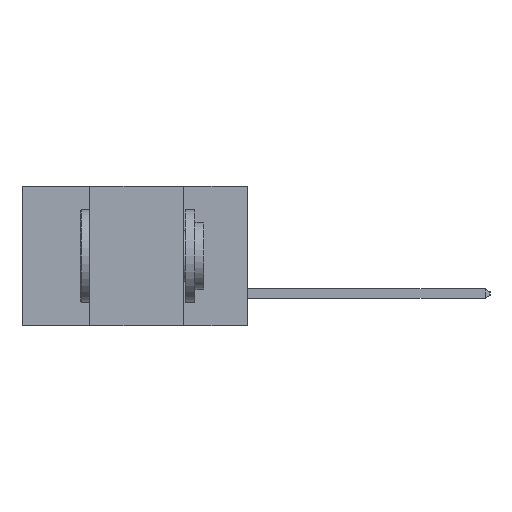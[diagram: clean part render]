
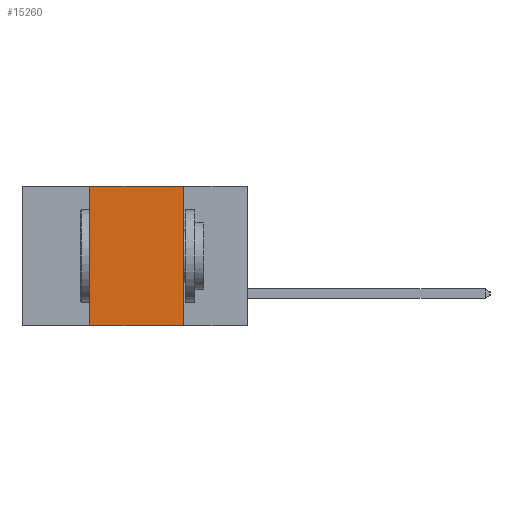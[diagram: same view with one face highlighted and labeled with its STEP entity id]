
A CAD part, left-side view. The second image highlights one B-rep face of the part: STEP entity #15260.
In plain terms, the highlighted planar face has unit normal (-1, 0, 0).
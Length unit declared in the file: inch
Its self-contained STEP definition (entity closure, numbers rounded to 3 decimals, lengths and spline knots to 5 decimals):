
#165 = CARTESIAN_POINT ( 'NONE',  ( 0., 0.6, -0.37 ) ) ;
#484 = CARTESIAN_POINT ( 'NONE',  ( 0., 0.42, -0.37 ) ) ;
#846 = CARTESIAN_POINT ( 'NONE',  ( 0., 0.6, 0. ) ) ;
#997 = VERTEX_POINT ( 'NONE', #6950 ) ;
#1227 = FACE_OUTER_BOUND ( 'NONE', #2528, .T. ) ;
#1617 = DIRECTION ( 'NONE',  ( 0., 0., -1. ) ) ;
#2177 = DIRECTION ( 'NONE',  ( 0., 0., -1. ) ) ;
#2320 = VERTEX_POINT ( 'NONE', #14089 ) ;
#2423 = DIRECTION ( 'NONE',  ( 0., -1., 0. ) ) ;
#2528 = EDGE_LOOP ( 'NONE', ( #11863, #14733, #8106, #14345 ) ) ;
#3344 = CARTESIAN_POINT ( 'NONE',  ( 0., 0.17, 0. ) ) ;
#6248 = CARTESIAN_POINT ( 'NONE',  ( 0., 0.6, 0. ) ) ;
#6489 = AXIS2_PLACEMENT_3D ( 'NONE', #846, #9815, #2177 ) ;
#6950 = CARTESIAN_POINT ( 'NONE',  ( 0., 0.42, 0. ) ) ;
#7304 = EDGE_CURVE ( 'NONE', #997, #10153, #13862, .T. ) ;
#7731 = VECTOR ( 'NONE', #1617, 39.37008 ) ;
#7892 = DIRECTION ( 'NONE',  ( 0., -1., 0. ) ) ;
#8106 = ORIENTED_EDGE ( 'NONE', *, *, #13539, .F. ) ;
#8115 = VECTOR ( 'NONE', #7892, 39.37008 ) ;
#8904 = LINE ( 'NONE', #12374, #15479 ) ;
#9255 = CARTESIAN_POINT ( 'NONE',  ( 0., 0.17, -0.37 ) ) ;
#9333 = VERTEX_POINT ( 'NONE', #484 ) ;
#9815 = DIRECTION ( 'NONE',  ( 1., 0., 0. ) ) ;
#10153 = VERTEX_POINT ( 'NONE', #3344 ) ;
#10701 = LINE ( 'NONE', #9255, #7731 ) ;
#11863 = ORIENTED_EDGE ( 'NONE', *, *, #12558, .F. ) ;
#12374 = CARTESIAN_POINT ( 'NONE',  ( 0., 0.42, -0.37 ) ) ;
#12521 = EDGE_CURVE ( 'NONE', #9333, #2320, #14742, .T. ) ;
#12558 = EDGE_CURVE ( 'NONE', #10153, #2320, #10701, .T. ) ;
#13092 = VECTOR ( 'NONE', #2423, 39.37008 ) ;
#13539 = EDGE_CURVE ( 'NONE', #9333, #997, #8904, .T. ) ;
#13591 = DIRECTION ( 'NONE',  ( 0., 0., 1. ) ) ;
#13862 = LINE ( 'NONE', #6248, #13092 ) ;
#14089 = CARTESIAN_POINT ( 'NONE',  ( 0., 0.17, -0.37 ) ) ;
#14345 = ORIENTED_EDGE ( 'NONE', *, *, #12521, .T. ) ;
#14733 = ORIENTED_EDGE ( 'NONE', *, *, #7304, .F. ) ;
#14739 = PLANE ( 'NONE',  #6489 ) ;
#14742 = LINE ( 'NONE', #165, #8115 ) ;
#15260 = ADVANCED_FACE ( 'NONE', ( #1227 ), #14739, .F. ) ;
#15479 = VECTOR ( 'NONE', #13591, 39.37008 ) ;
